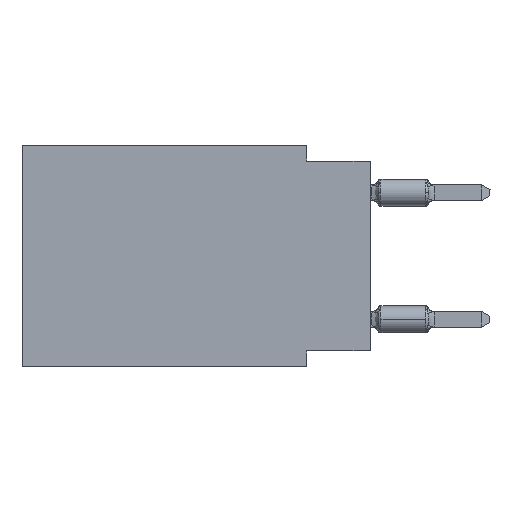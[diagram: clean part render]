
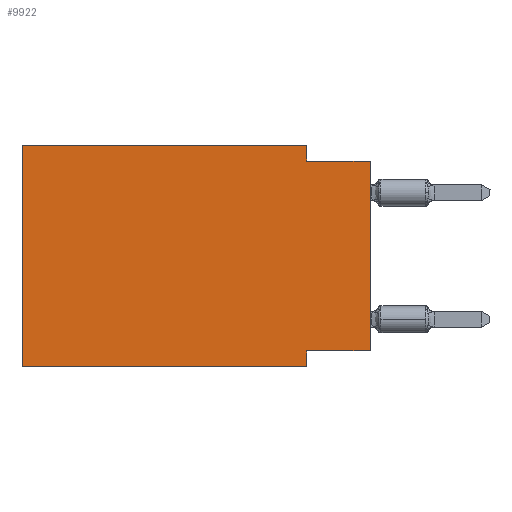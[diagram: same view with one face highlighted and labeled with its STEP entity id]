
A CAD part, left-side view. The second image highlights one B-rep face of the part: STEP entity #9922.
In plain terms, the highlighted planar face has unit normal (-1, 0, 0).
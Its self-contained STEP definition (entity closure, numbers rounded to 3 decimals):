
#21 = LINE ( 'NONE', #9247, #11440 ) ;
#497 = EDGE_LOOP ( 'NONE', ( #18333, #10147, #13976, #22274, #17851, #21935, #24459, #22683 ) ) ;
#694 = VECTOR ( 'NONE', #1341, 1000. ) ;
#714 = DIRECTION ( 'NONE',  ( 0., 0., -1. ) ) ;
#939 = EDGE_CURVE ( 'NONE', #12149, #20092, #21, .T. ) ;
#1341 = DIRECTION ( 'NONE',  ( 0., -1., 0. ) ) ;
#1567 = EDGE_CURVE ( 'NONE', #4986, #12149, #10333, .T. ) ;
#1938 = VECTOR ( 'NONE', #4016, 1000. ) ;
#1968 = LINE ( 'NONE', #21408, #2756 ) ;
#2009 = CARTESIAN_POINT ( 'NONE',  ( 0., 0., -8.255 ) ) ;
#2299 = VECTOR ( 'NONE', #20056, 1000. ) ;
#2398 = EDGE_CURVE ( 'NONE', #21228, #4986, #7332, .T. ) ;
#2506 = VERTEX_POINT ( 'NONE', #2009 ) ;
#2756 = VECTOR ( 'NONE', #19509, 1000. ) ;
#3608 = CARTESIAN_POINT ( 'NONE',  ( 0., 2.54, -8.89 ) ) ;
#4016 = DIRECTION ( 'NONE',  ( 0., 0., 1. ) ) ;
#4611 = LINE ( 'NONE', #12571, #1938 ) ;
#4695 = CARTESIAN_POINT ( 'NONE',  ( 0., 2.54, -0.635 ) ) ;
#4986 = VERTEX_POINT ( 'NONE', #16150 ) ;
#5004 = CARTESIAN_POINT ( 'NONE',  ( 0., 13.97, -8.89 ) ) ;
#5034 = VERTEX_POINT ( 'NONE', #7172 ) ;
#5130 = LINE ( 'NONE', #5004, #694 ) ;
#5451 = PLANE ( 'NONE',  #19132 ) ;
#6877 = VERTEX_POINT ( 'NONE', #3608 ) ;
#7172 = CARTESIAN_POINT ( 'NONE',  ( 0., 13.97, -8.89 ) ) ;
#7332 = LINE ( 'NONE', #11374, #16499 ) ;
#7468 = DIRECTION ( 'NONE',  ( 0., 0., -1. ) ) ;
#7577 = DIRECTION ( 'NONE',  ( 0., -1., 0. ) ) ;
#8268 = CARTESIAN_POINT ( 'NONE',  ( 0., 0., -0.635 ) ) ;
#8293 = LINE ( 'NONE', #14221, #13414 ) ;
#9247 = CARTESIAN_POINT ( 'NONE',  ( 0., 0., -0.635 ) ) ;
#9922 = ADVANCED_FACE ( 'NONE', ( #15036 ), #5451, .F. ) ;
#10147 = ORIENTED_EDGE ( 'NONE', *, *, #939, .F. ) ;
#10333 = LINE ( 'NONE', #22417, #12032 ) ;
#10578 = CARTESIAN_POINT ( 'NONE',  ( 0., 2.54, -8.255 ) ) ;
#10710 = CARTESIAN_POINT ( 'NONE',  ( 0., 0., 0. ) ) ;
#11374 = CARTESIAN_POINT ( 'NONE',  ( 0., 13.97, 0. ) ) ;
#11440 = VECTOR ( 'NONE', #16817, 1000. ) ;
#12032 = VECTOR ( 'NONE', #14705, 1000. ) ;
#12149 = VERTEX_POINT ( 'NONE', #4695 ) ;
#12414 = EDGE_CURVE ( 'NONE', #22660, #6877, #8293, .T. ) ;
#12571 = CARTESIAN_POINT ( 'NONE',  ( 0., 13.97, 0. ) ) ;
#13146 = CARTESIAN_POINT ( 'NONE',  ( 0., 13.97, 0. ) ) ;
#13414 = VECTOR ( 'NONE', #714, 1000. ) ;
#13976 = ORIENTED_EDGE ( 'NONE', *, *, #1567, .F. ) ;
#14221 = CARTESIAN_POINT ( 'NONE',  ( 0., 2.54, -8.89 ) ) ;
#14705 = DIRECTION ( 'NONE',  ( 0., 0., -1. ) ) ;
#15036 = FACE_OUTER_BOUND ( 'NONE', #497, .T. ) ;
#15891 = LINE ( 'NONE', #10710, #2299 ) ;
#16150 = CARTESIAN_POINT ( 'NONE',  ( 0., 2.54, 0. ) ) ;
#16499 = VECTOR ( 'NONE', #7577, 1000. ) ;
#16817 = DIRECTION ( 'NONE',  ( 0., -1., 0. ) ) ;
#17851 = ORIENTED_EDGE ( 'NONE', *, *, #21361, .F. ) ;
#18333 = ORIENTED_EDGE ( 'NONE', *, *, #24601, .T. ) ;
#19130 = EDGE_CURVE ( 'NONE', #5034, #6877, #5130, .T. ) ;
#19132 = AXIS2_PLACEMENT_3D ( 'NONE', #13146, #20844, #7468 ) ;
#19175 = CARTESIAN_POINT ( 'NONE',  ( 0., 13.97, 0. ) ) ;
#19509 = DIRECTION ( 'NONE',  ( 0., 1., 0. ) ) ;
#20001 = EDGE_CURVE ( 'NONE', #2506, #22660, #1968, .T. ) ;
#20056 = DIRECTION ( 'NONE',  ( 0., 0., 1. ) ) ;
#20092 = VERTEX_POINT ( 'NONE', #8268 ) ;
#20844 = DIRECTION ( 'NONE',  ( 1., 0., 0. ) ) ;
#21228 = VERTEX_POINT ( 'NONE', #19175 ) ;
#21361 = EDGE_CURVE ( 'NONE', #5034, #21228, #4611, .T. ) ;
#21408 = CARTESIAN_POINT ( 'NONE',  ( 0., 0., -8.255 ) ) ;
#21935 = ORIENTED_EDGE ( 'NONE', *, *, #19130, .T. ) ;
#22274 = ORIENTED_EDGE ( 'NONE', *, *, #2398, .F. ) ;
#22417 = CARTESIAN_POINT ( 'NONE',  ( 0., 2.54, 0. ) ) ;
#22660 = VERTEX_POINT ( 'NONE', #10578 ) ;
#22683 = ORIENTED_EDGE ( 'NONE', *, *, #20001, .F. ) ;
#24459 = ORIENTED_EDGE ( 'NONE', *, *, #12414, .F. ) ;
#24601 = EDGE_CURVE ( 'NONE', #2506, #20092, #15891, .T. ) ;
